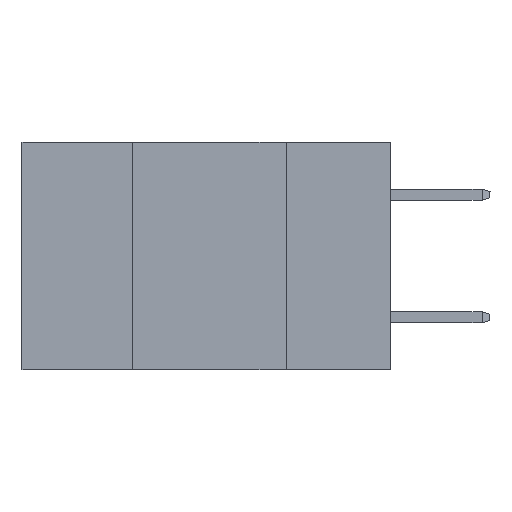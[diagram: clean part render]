
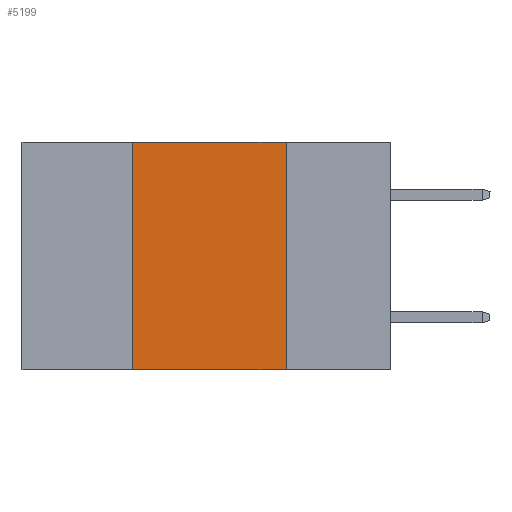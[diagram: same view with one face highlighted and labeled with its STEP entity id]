
A CAD part, left-side view. The second image highlights one B-rep face of the part: STEP entity #5199.
In plain terms, the highlighted planar face has unit normal (-1, 0, 0).
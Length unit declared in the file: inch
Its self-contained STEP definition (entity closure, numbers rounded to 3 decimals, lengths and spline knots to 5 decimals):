
#391 = CARTESIAN_POINT ( 'NONE',  ( 0., 0.17, 0. ) ) ;
#1160 = ORIENTED_EDGE ( 'NONE', *, *, #15672, .F. ) ;
#1684 = DIRECTION ( 'NONE',  ( 0., -1., 0. ) ) ;
#2410 = CARTESIAN_POINT ( 'NONE',  ( 0., 0.17, -0.37 ) ) ;
#2637 = EDGE_CURVE ( 'NONE', #4229, #6118, #6942, .T. ) ;
#2716 = DIRECTION ( 'NONE',  ( 0., 0., -1. ) ) ;
#3047 = DIRECTION ( 'NONE',  ( 0., 0., 1. ) ) ;
#4229 = VERTEX_POINT ( 'NONE', #7634 ) ;
#4833 = VECTOR ( 'NONE', #1684, 39.37008 ) ;
#5105 = CARTESIAN_POINT ( 'NONE',  ( 0., 0.17, 0. ) ) ;
#5116 = ORIENTED_EDGE ( 'NONE', *, *, #2637, .T. ) ;
#5130 = EDGE_LOOP ( 'NONE', ( #1160, #5171, #6660, #5116 ) ) ;
#5171 = ORIENTED_EDGE ( 'NONE', *, *, #9622, .F. ) ;
#5199 = ADVANCED_FACE ( 'NONE', ( #8366 ), #16150, .F. ) ;
#5867 = CARTESIAN_POINT ( 'NONE',  ( 0., 0.6, -0.37 ) ) ;
#6118 = VERTEX_POINT ( 'NONE', #2410 ) ;
#6168 = VECTOR ( 'NONE', #15685, 39.37008 ) ;
#6660 = ORIENTED_EDGE ( 'NONE', *, *, #12994, .F. ) ;
#6942 = LINE ( 'NONE', #5867, #6168 ) ;
#7634 = CARTESIAN_POINT ( 'NONE',  ( 0., 0.42, -0.37 ) ) ;
#7639 = DIRECTION ( 'NONE',  ( 1., 0., 0. ) ) ;
#7787 = DIRECTION ( 'NONE',  ( 0., 0., -1. ) ) ;
#8366 = FACE_OUTER_BOUND ( 'NONE', #5130, .T. ) ;
#9622 = EDGE_CURVE ( 'NONE', #11254, #10053, #10261, .T. ) ;
#10053 = VERTEX_POINT ( 'NONE', #391 ) ;
#10261 = LINE ( 'NONE', #15254, #4833 ) ;
#10701 = VECTOR ( 'NONE', #7787, 39.37008 ) ;
#11243 = CARTESIAN_POINT ( 'NONE',  ( 0., 0.6, 0. ) ) ;
#11254 = VERTEX_POINT ( 'NONE', #14200 ) ;
#11802 = CARTESIAN_POINT ( 'NONE',  ( 0., 0.42, 0. ) ) ;
#12994 = EDGE_CURVE ( 'NONE', #4229, #11254, #15852, .T. ) ;
#13065 = LINE ( 'NONE', #5105, #10701 ) ;
#13934 = AXIS2_PLACEMENT_3D ( 'NONE', #11243, #7639, #2716 ) ;
#14200 = CARTESIAN_POINT ( 'NONE',  ( 0., 0.42, 0. ) ) ;
#15254 = CARTESIAN_POINT ( 'NONE',  ( 0., 0.6, 0. ) ) ;
#15298 = VECTOR ( 'NONE', #3047, 39.37008 ) ;
#15672 = EDGE_CURVE ( 'NONE', #10053, #6118, #13065, .T. ) ;
#15685 = DIRECTION ( 'NONE',  ( 0., -1., 0. ) ) ;
#15852 = LINE ( 'NONE', #11802, #15298 ) ;
#16150 = PLANE ( 'NONE',  #13934 ) ;
